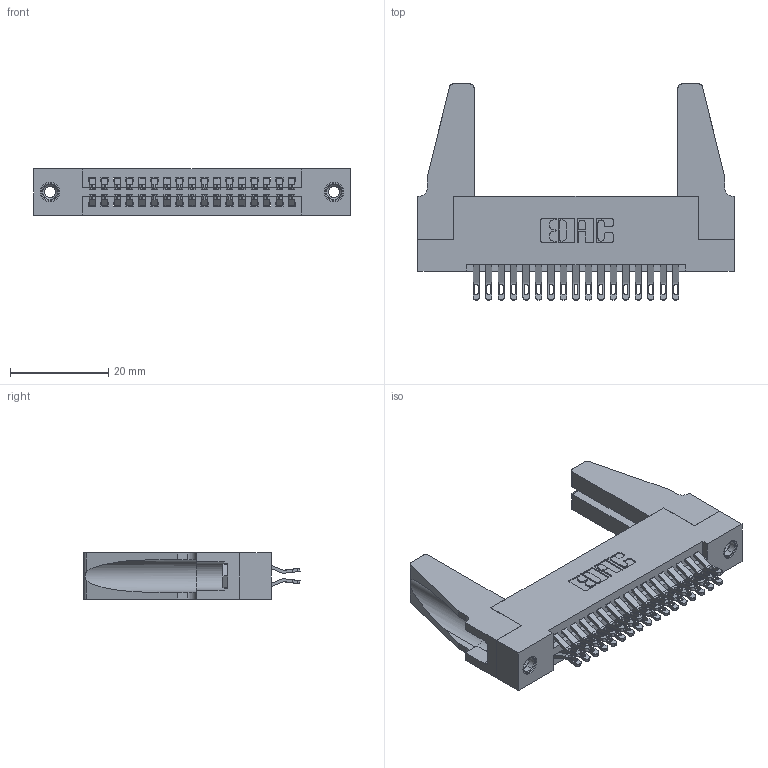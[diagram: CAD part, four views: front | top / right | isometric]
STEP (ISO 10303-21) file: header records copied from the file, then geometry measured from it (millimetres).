
FILE_DESCRIPTION (( 'STEP AP203' ), '1' );
FILE_NAME ('395-034-555-288.STEP', '2019-10-17T18:10:07', ( '' ), ( '' ), 'SwSTEP 2.0', 'SolidWorks 2016', '' );
FILE_SCHEMA (( 'CONFIG_CONTROL_DESIGN' ));
Length unit declared in the file: inch
Products named in the file (5): 395-034-555-288; 345 Part_Flush Mounting Lugs - 0.156 Dia-TH; 345-292-001_555 Tail; 345-250-001_345-250-001-102; 345-220-078_345-220-088
Assembly tree (39 placements, depth 2):
  395-034-555-288
    345 Part_Flush Mounting Lugs - 0.156 Dia-TH
    345-292-001_555 Tail  x34
    345-250-001_345-250-001-102  x2
    345-220-078_345-220-088  x2
Bounding box: 64.41 x 43.99 x 9.4 mm (x, y, z)
Volume: 9376.3 mm3; surface area: 12033 mm2
Topology: 39 solids, 39 shells, 2154 faces, 6673 edges, 4438 vertices
Faces by surface type: plane 1206, cylinder 932, cone 12, torus 4
Entity records: 19178 total; most frequent: CARTESIAN_POINT 3268, ORIENTED_EDGE 3132, DIRECTION 2886, EDGE_CURVE 1566, VECTOR 1304, LINE 1304, VERTEX_POINT 1038, AXIS2_PLACEMENT_3D 791
